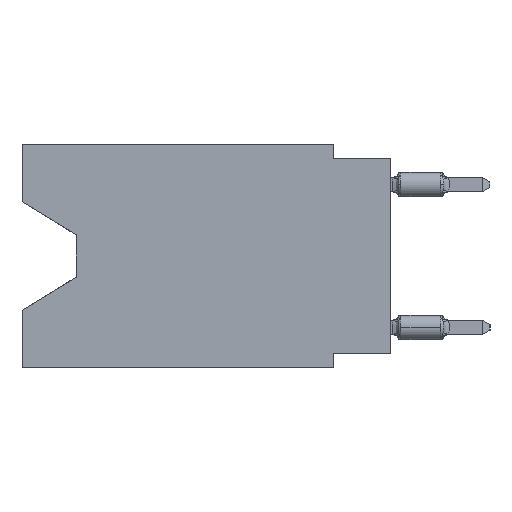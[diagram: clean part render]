
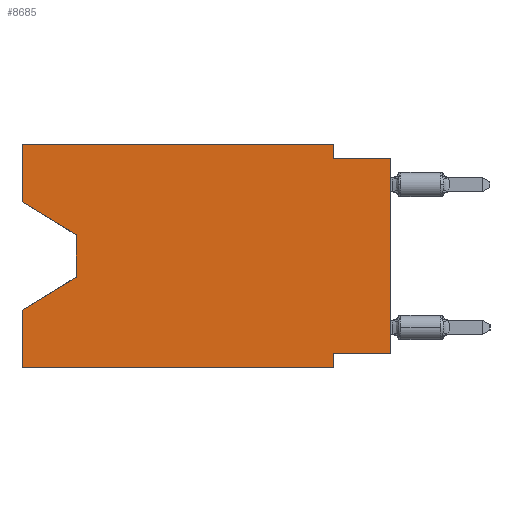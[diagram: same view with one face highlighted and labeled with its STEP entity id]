
A CAD part, left-side view. The second image highlights one B-rep face of the part: STEP entity #8685.
In plain terms, the highlighted planar face has unit normal (-1, 0, 0).
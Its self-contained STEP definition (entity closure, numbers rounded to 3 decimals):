
#215 = ORIENTED_EDGE ( 'NONE', *, *, #13867, .T. ) ;
#607 = DIRECTION ( 'NONE',  ( 0., 0., 1. ) ) ;
#647 = EDGE_CURVE ( 'NONE', #8970, #32543, #32854, .T. ) ;
#1456 = VERTEX_POINT ( 'NONE', #12260 ) ;
#1488 = EDGE_CURVE ( 'NONE', #27177, #34065, #3247, .T. ) ;
#1775 = CARTESIAN_POINT ( 'NONE',  ( 0., 16.383, -9.906 ) ) ;
#2040 = VERTEX_POINT ( 'NONE', #32194 ) ;
#2346 = VECTOR ( 'NONE', #29659, 1000. ) ;
#3151 = LINE ( 'NONE', #31053, #27236 ) ;
#3247 = LINE ( 'NONE', #18181, #14272 ) ;
#3544 = EDGE_LOOP ( 'NONE', ( #3847, #19721, #33078, #9117, #215, #25396, #31388, #28836, #36301, #32544, #36356, #33890 ) ) ;
#3838 = VECTOR ( 'NONE', #20938, 1000. ) ;
#3847 = ORIENTED_EDGE ( 'NONE', *, *, #9178, .T. ) ;
#4038 = CARTESIAN_POINT ( 'NONE',  ( 0., 16.383, 0. ) ) ;
#4955 = DIRECTION ( 'NONE',  ( 0., 0., 1. ) ) ;
#5063 = VERTEX_POINT ( 'NONE', #1775 ) ;
#5085 = VECTOR ( 'NONE', #6878, 1000. ) ;
#5220 = LINE ( 'NONE', #16611, #3838 ) ;
#5370 = EDGE_CURVE ( 'NONE', #5063, #1456, #32414, .T. ) ;
#6744 = CARTESIAN_POINT ( 'NONE',  ( 0., 16.383, 0. ) ) ;
#6878 = DIRECTION ( 'NONE',  ( 0., 1., 0. ) ) ;
#7721 = FACE_OUTER_BOUND ( 'NONE', #3544, .T. ) ;
#8487 = LINE ( 'NONE', #20258, #23951 ) ;
#8685 = ADVANCED_FACE ( 'NONE', ( #7721 ), #10323, .F. ) ;
#8970 = VERTEX_POINT ( 'NONE', #6744 ) ;
#9117 = ORIENTED_EDGE ( 'NONE', *, *, #5370, .F. ) ;
#9178 = EDGE_CURVE ( 'NONE', #33633, #27788, #8487, .T. ) ;
#9738 = LINE ( 'NONE', #15919, #27345 ) ;
#9787 = CARTESIAN_POINT ( 'NONE',  ( 0., 16.383, -9.906 ) ) ;
#9896 = CARTESIAN_POINT ( 'NONE',  ( 0., 2.54, -9.271 ) ) ;
#10323 = PLANE ( 'NONE',  #14985 ) ;
#10707 = DIRECTION ( 'NONE',  ( 0., 0., -1. ) ) ;
#10751 = LINE ( 'NONE', #36202, #28902 ) ;
#11237 = CARTESIAN_POINT ( 'NONE',  ( 0., 2.54, 0. ) ) ;
#11259 = EDGE_CURVE ( 'NONE', #32543, #18343, #20243, .T. ) ;
#11284 = DIRECTION ( 'NONE',  ( 0., 0., -1. ) ) ;
#11646 = CARTESIAN_POINT ( 'NONE',  ( 0., 2.54, 0. ) ) ;
#11847 = DIRECTION ( 'NONE',  ( 0., -0.855, -0.519 ) ) ;
#12260 = CARTESIAN_POINT ( 'NONE',  ( 0., 16.383, -7.36 ) ) ;
#12650 = LINE ( 'NONE', #26684, #5085 ) ;
#12771 = CARTESIAN_POINT ( 'NONE',  ( 0., 16.383, 0. ) ) ;
#12982 = CARTESIAN_POINT ( 'NONE',  ( 0., 0., -9.271 ) ) ;
#13029 = CARTESIAN_POINT ( 'NONE',  ( 0., 0., 0. ) ) ;
#13867 = EDGE_CURVE ( 'NONE', #5063, #34065, #23975, .T. ) ;
#13966 = VERTEX_POINT ( 'NONE', #12982 ) ;
#14272 = VECTOR ( 'NONE', #26054, 1000. ) ;
#14968 = EDGE_CURVE ( 'NONE', #18343, #36302, #5220, .T. ) ;
#14985 = AXIS2_PLACEMENT_3D ( 'NONE', #19109, #16302, #10707 ) ;
#15726 = DIRECTION ( 'NONE',  ( 0., 0., -1. ) ) ;
#15919 = CARTESIAN_POINT ( 'NONE',  ( 0., 13.97, -4.013 ) ) ;
#16258 = EDGE_CURVE ( 'NONE', #13966, #36302, #30041, .T. ) ;
#16302 = DIRECTION ( 'NONE',  ( 1., 0., 0. ) ) ;
#16338 = VECTOR ( 'NONE', #17836, 1000. ) ;
#16611 = CARTESIAN_POINT ( 'NONE',  ( 0., 0., -0.635 ) ) ;
#17728 = CARTESIAN_POINT ( 'NONE',  ( 0., 0., -0.635 ) ) ;
#17754 = VECTOR ( 'NONE', #11284, 1000. ) ;
#17836 = DIRECTION ( 'NONE',  ( 0., -1., 0. ) ) ;
#18181 = CARTESIAN_POINT ( 'NONE',  ( 0., 2.54, -9.906 ) ) ;
#18343 = VERTEX_POINT ( 'NONE', #34984 ) ;
#19109 = CARTESIAN_POINT ( 'NONE',  ( 0., 16.383, 0. ) ) ;
#19721 = ORIENTED_EDGE ( 'NONE', *, *, #32363, .T. ) ;
#20243 = LINE ( 'NONE', #11646, #17754 ) ;
#20258 = CARTESIAN_POINT ( 'NONE',  ( 0., 16.383, -2.546 ) ) ;
#20700 = EDGE_CURVE ( 'NONE', #33633, #8970, #10751, .T. ) ;
#20938 = DIRECTION ( 'NONE',  ( 0., -1., 0. ) ) ;
#23052 = CARTESIAN_POINT ( 'NONE',  ( 0., 13.97, -4.013 ) ) ;
#23394 = EDGE_CURVE ( 'NONE', #13966, #27177, #12650, .T. ) ;
#23951 = VECTOR ( 'NONE', #11847, 1000. ) ;
#23975 = LINE ( 'NONE', #9787, #16338 ) ;
#24819 = VECTOR ( 'NONE', #30424, 1000. ) ;
#25396 = ORIENTED_EDGE ( 'NONE', *, *, #1488, .F. ) ;
#25967 = DIRECTION ( 'NONE',  ( 0., 0.855, -0.519 ) ) ;
#26054 = DIRECTION ( 'NONE',  ( 0., 0., -1. ) ) ;
#26684 = CARTESIAN_POINT ( 'NONE',  ( 0., 0., -9.271 ) ) ;
#27177 = VERTEX_POINT ( 'NONE', #9896 ) ;
#27236 = VECTOR ( 'NONE', #25967, 1000. ) ;
#27345 = VECTOR ( 'NONE', #15726, 1000. ) ;
#27788 = VERTEX_POINT ( 'NONE', #23052 ) ;
#27796 = CARTESIAN_POINT ( 'NONE',  ( 0., 16.383, -2.546 ) ) ;
#28836 = ORIENTED_EDGE ( 'NONE', *, *, #16258, .T. ) ;
#28902 = VECTOR ( 'NONE', #4955, 1000. ) ;
#29659 = DIRECTION ( 'NONE',  ( 0., -1., 0. ) ) ;
#30041 = LINE ( 'NONE', #13029, #24819 ) ;
#30424 = DIRECTION ( 'NONE',  ( 0., 0., 1. ) ) ;
#31053 = CARTESIAN_POINT ( 'NONE',  ( 0., 13.97, -5.893 ) ) ;
#31388 = ORIENTED_EDGE ( 'NONE', *, *, #23394, .F. ) ;
#31787 = VECTOR ( 'NONE', #607, 1000. ) ;
#32194 = CARTESIAN_POINT ( 'NONE',  ( 0., 13.97, -5.893 ) ) ;
#32363 = EDGE_CURVE ( 'NONE', #27788, #2040, #9738, .T. ) ;
#32414 = LINE ( 'NONE', #12771, #31787 ) ;
#32543 = VERTEX_POINT ( 'NONE', #11237 ) ;
#32544 = ORIENTED_EDGE ( 'NONE', *, *, #11259, .F. ) ;
#32854 = LINE ( 'NONE', #4038, #2346 ) ;
#33078 = ORIENTED_EDGE ( 'NONE', *, *, #36908, .T. ) ;
#33633 = VERTEX_POINT ( 'NONE', #27796 ) ;
#33890 = ORIENTED_EDGE ( 'NONE', *, *, #20700, .F. ) ;
#34065 = VERTEX_POINT ( 'NONE', #34118 ) ;
#34118 = CARTESIAN_POINT ( 'NONE',  ( 0., 2.54, -9.906 ) ) ;
#34984 = CARTESIAN_POINT ( 'NONE',  ( 0., 2.54, -0.635 ) ) ;
#36202 = CARTESIAN_POINT ( 'NONE',  ( 0., 16.383, 0. ) ) ;
#36301 = ORIENTED_EDGE ( 'NONE', *, *, #14968, .F. ) ;
#36302 = VERTEX_POINT ( 'NONE', #17728 ) ;
#36356 = ORIENTED_EDGE ( 'NONE', *, *, #647, .F. ) ;
#36908 = EDGE_CURVE ( 'NONE', #2040, #1456, #3151, .T. ) ;
